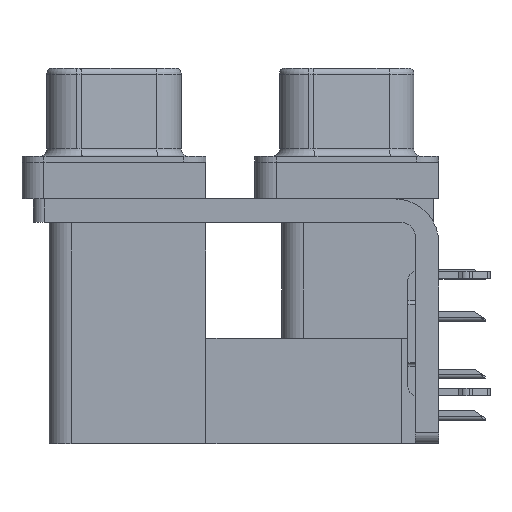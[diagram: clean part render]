
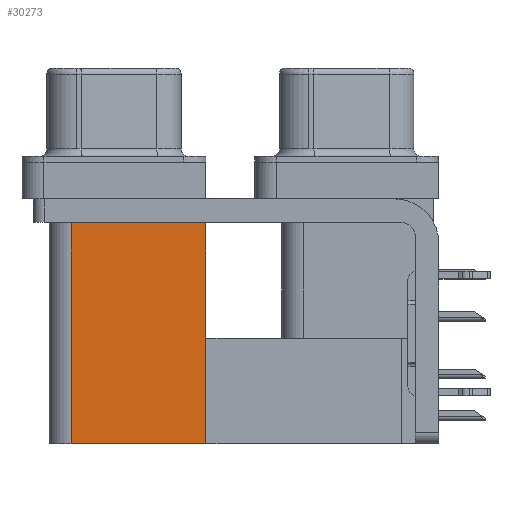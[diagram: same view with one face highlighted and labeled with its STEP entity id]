
A CAD part, left-side view. The second image highlights one B-rep face of the part: STEP entity #30273.
In plain terms, the highlighted planar face has unit normal (-1, 0, 0).
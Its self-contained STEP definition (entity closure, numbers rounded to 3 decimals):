
#254 = CARTESIAN_POINT ( 'NONE',  ( 3.765, 9.6, -19.2 ) ) ;
#3294 = VECTOR ( 'NONE', #33194, 1000. ) ;
#4093 = CARTESIAN_POINT ( 'NONE',  ( 3.765, 9.6, -19.2 ) ) ;
#5694 = EDGE_LOOP ( 'NONE', ( #18261, #12564, #26318, #9268 ) ) ;
#6429 = DIRECTION ( 'NONE',  ( 0., 1., 0. ) ) ;
#6833 = DIRECTION ( 'NONE',  ( 1., 0., 0. ) ) ;
#9268 = ORIENTED_EDGE ( 'NONE', *, *, #16724, .T. ) ;
#9391 = FACE_OUTER_BOUND ( 'NONE', #5694, .T. ) ;
#9656 = AXIS2_PLACEMENT_3D ( 'NONE', #19893, #6833, #17317 ) ;
#11756 = CARTESIAN_POINT ( 'NONE',  ( 3.765, 9.6, -2.5 ) ) ;
#12564 = ORIENTED_EDGE ( 'NONE', *, *, #16709, .F. ) ;
#14118 = VERTEX_POINT ( 'NONE', #22202 ) ;
#14959 = LINE ( 'NONE', #17551, #3294 ) ;
#15192 = EDGE_CURVE ( 'NONE', #20561, #14118, #17154, .T. ) ;
#15360 = DIRECTION ( 'NONE',  ( 0., 1., 0. ) ) ;
#15459 = LINE ( 'NONE', #20619, #28097 ) ;
#16709 = EDGE_CURVE ( 'NONE', #14118, #20465, #14959, .T. ) ;
#16724 = EDGE_CURVE ( 'NONE', #20561, #17421, #15459, .T. ) ;
#17154 = LINE ( 'NONE', #4093, #24156 ) ;
#17280 = VECTOR ( 'NONE', #6429, 1000. ) ;
#17317 = DIRECTION ( 'NONE',  ( 0., 0., -1. ) ) ;
#17421 = VERTEX_POINT ( 'NONE', #26753 ) ;
#17551 = CARTESIAN_POINT ( 'NONE',  ( 3.765, 18.8, -19.2 ) ) ;
#18261 = ORIENTED_EDGE ( 'NONE', *, *, #29023, .T. ) ;
#19663 = LINE ( 'NONE', #11756, #17280 ) ;
#19893 = CARTESIAN_POINT ( 'NONE',  ( 3.765, 9.6, -19.2 ) ) ;
#20465 = VERTEX_POINT ( 'NONE', #23791 ) ;
#20561 = VERTEX_POINT ( 'NONE', #254 ) ;
#20619 = CARTESIAN_POINT ( 'NONE',  ( 3.765, 9.6, -19.2 ) ) ;
#22202 = CARTESIAN_POINT ( 'NONE',  ( 3.765, 18.8, -19.2 ) ) ;
#23791 = CARTESIAN_POINT ( 'NONE',  ( 3.765, 18.8, -2.5 ) ) ;
#24156 = VECTOR ( 'NONE', #15360, 1000. ) ;
#26318 = ORIENTED_EDGE ( 'NONE', *, *, #15192, .F. ) ;
#26753 = CARTESIAN_POINT ( 'NONE',  ( 3.765, 9.6, -2.5 ) ) ;
#28097 = VECTOR ( 'NONE', #31118, 1000. ) ;
#29023 = EDGE_CURVE ( 'NONE', #17421, #20465, #19663, .T. ) ;
#30273 = ADVANCED_FACE ( 'NONE', ( #9391 ), #32952, .F. ) ;
#31118 = DIRECTION ( 'NONE',  ( 0., 0., 1. ) ) ;
#32952 = PLANE ( 'NONE',  #9656 ) ;
#33194 = DIRECTION ( 'NONE',  ( 0., 0., 1. ) ) ;
